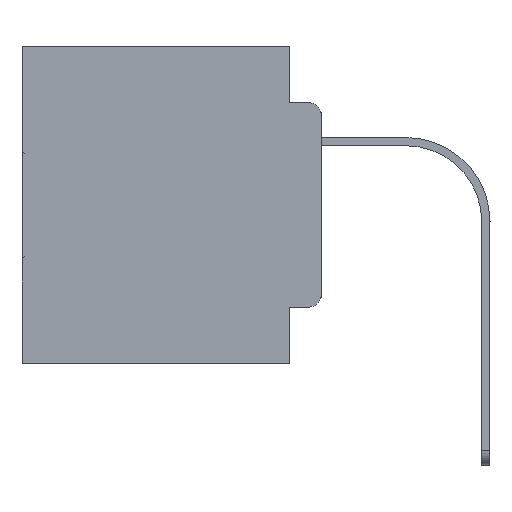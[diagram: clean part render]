
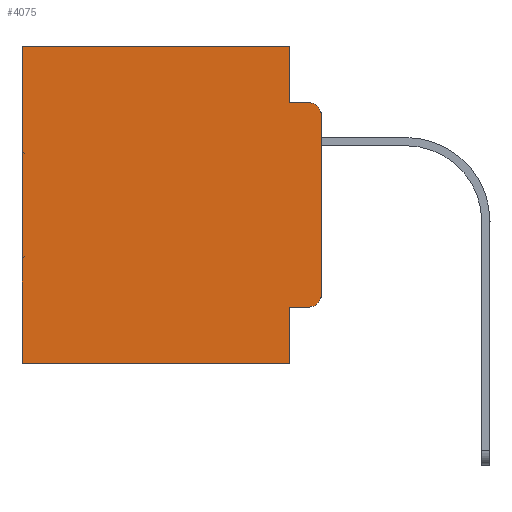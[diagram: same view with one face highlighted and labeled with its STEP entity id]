
A CAD part, left-side view. The second image highlights one B-rep face of the part: STEP entity #4075.
In plain terms, the highlighted planar face has unit normal (-1, 0, 0).
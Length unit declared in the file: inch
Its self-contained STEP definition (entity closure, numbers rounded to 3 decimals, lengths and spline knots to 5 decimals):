
#538 = VERTEX_POINT ( 'NONE', #17069 ) ;
#594 = CARTESIAN_POINT ( 'NONE',  ( 0.298, 0.473, 0. ) ) ;
#929 = DIRECTION ( 'NONE',  ( 0., 0., -1. ) ) ;
#1005 = CARTESIAN_POINT ( 'NONE',  ( 0.298, 0., 0. ) ) ;
#1598 = EDGE_CURVE ( 'NONE', #16262, #1641, #28964, .T. ) ;
#1641 = VERTEX_POINT ( 'NONE', #12351 ) ;
#2139 = LINE ( 'NONE', #21336, #22587 ) ;
#3368 = DIRECTION ( 'NONE',  ( 1., 0., 0. ) ) ;
#3558 = ORIENTED_EDGE ( 'NONE', *, *, #11707, .F. ) ;
#3778 = ORIENTED_EDGE ( 'NONE', *, *, #1598, .F. ) ;
#4075 = ADVANCED_FACE ( 'NONE', ( #20603 ), #30549, .F. ) ;
#4396 = CARTESIAN_POINT ( 'NONE',  ( 0.298, 0.051, 0. ) ) ;
#4466 = VERTEX_POINT ( 'NONE', #18658 ) ;
#6388 = EDGE_CURVE ( 'NONE', #16262, #13022, #28228, .T. ) ;
#6582 = CARTESIAN_POINT ( 'NONE',  ( 0.298, 0., -0.1085 ) ) ;
#8537 = CARTESIAN_POINT ( 'NONE',  ( 0.298, 0.051, 0. ) ) ;
#8723 = ORIENTED_EDGE ( 'NONE', *, *, #19751, .T. ) ;
#8855 = CARTESIAN_POINT ( 'NONE',  ( 0.298, 0., 0. ) ) ;
#9914 = VECTOR ( 'NONE', #22390, 39.37008 ) ;
#10277 = DIRECTION ( 'NONE',  ( 0., 0., -1. ) ) ;
#10423 = DIRECTION ( 'NONE',  ( -1., 0., 0. ) ) ;
#10648 = ORIENTED_EDGE ( 'NONE', *, *, #12283, .F. ) ;
#10711 = LINE ( 'NONE', #594, #16738 ) ;
#10853 = CARTESIAN_POINT ( 'NONE',  ( 0.298, 0., 0. ) ) ;
#11054 = CARTESIAN_POINT ( 'NONE',  ( 0.298, 0.02, -0.1085 ) ) ;
#11199 = CARTESIAN_POINT ( 'NONE',  ( 0.298, 0.473, 0. ) ) ;
#11707 = EDGE_CURVE ( 'NONE', #1641, #31300, #23032, .T. ) ;
#11749 = ORIENTED_EDGE ( 'NONE', *, *, #12856, .T. ) ;
#11909 = ORIENTED_EDGE ( 'NONE', *, *, #29803, .F. ) ;
#12055 = ORIENTED_EDGE ( 'NONE', *, *, #15059, .T. ) ;
#12086 = DIRECTION ( 'NONE',  ( 0., 1., 0. ) ) ;
#12283 = EDGE_CURVE ( 'NONE', #4466, #26132, #13297, .T. ) ;
#12351 = CARTESIAN_POINT ( 'NONE',  ( 0.298, 0.051, -0.0885 ) ) ;
#12856 = EDGE_CURVE ( 'NONE', #13022, #26415, #10711, .T. ) ;
#13017 = CARTESIAN_POINT ( 'NONE',  ( 0.298, 0.02, -0.0885 ) ) ;
#13022 = VERTEX_POINT ( 'NONE', #11199 ) ;
#13297 = LINE ( 'NONE', #8537, #20169 ) ;
#14974 = ORIENTED_EDGE ( 'NONE', *, *, #29296, .T. ) ;
#15059 = EDGE_CURVE ( 'NONE', #31865, #31300, #25568, .T. ) ;
#15273 = CARTESIAN_POINT ( 'NONE',  ( 0.298, 0.051, -0.0885 ) ) ;
#16262 = VERTEX_POINT ( 'NONE', #4396 ) ;
#16738 = VECTOR ( 'NONE', #20138, 39.37008 ) ;
#17069 = CARTESIAN_POINT ( 'NONE',  ( 0.298, 0., -0.3915 ) ) ;
#17195 = CARTESIAN_POINT ( 'NONE',  ( 0.298, 0.051, 0. ) ) ;
#18249 = DIRECTION ( 'NONE',  ( 0., 0., -1. ) ) ;
#18477 = DIRECTION ( 'NONE',  ( 0., 0., -1. ) ) ;
#18566 = DIRECTION ( 'NONE',  ( 0., 0., -1. ) ) ;
#18658 = CARTESIAN_POINT ( 'NONE',  ( 0.298, 0.051, -0.4115 ) ) ;
#18780 = DIRECTION ( 'NONE',  ( 0., 1., 0. ) ) ;
#19317 = DIRECTION ( 'NONE',  ( 0., 0., -1. ) ) ;
#19751 = EDGE_CURVE ( 'NONE', #4466, #31774, #29927, .T. ) ;
#20138 = DIRECTION ( 'NONE',  ( 0., 0., -1. ) ) ;
#20169 = VECTOR ( 'NONE', #18477, 39.37008 ) ;
#20555 = VECTOR ( 'NONE', #29755, 39.37008 ) ;
#20603 = FACE_OUTER_BOUND ( 'NONE', #21703, .T. ) ;
#20965 = DIRECTION ( 'NONE',  ( -1., 0., 0. ) ) ;
#21018 = VECTOR ( 'NONE', #18780, 39.37008 ) ;
#21336 = CARTESIAN_POINT ( 'NONE',  ( 0.298, 0., -0.5 ) ) ;
#21703 = EDGE_LOOP ( 'NONE', ( #27954, #12055, #3558, #3778, #28477, #11749, #11909, #10648, #8723, #14974 ) ) ;
#21880 = AXIS2_PLACEMENT_3D ( 'NONE', #25393, #10423, #10277 ) ;
#22253 = CARTESIAN_POINT ( 'NONE',  ( 0.298, 0.051, -0.4115 ) ) ;
#22390 = DIRECTION ( 'NONE',  ( 0., -1., 0. ) ) ;
#22587 = VECTOR ( 'NONE', #12086, 39.37008 ) ;
#23032 = LINE ( 'NONE', #15273, #9914 ) ;
#24361 = EDGE_CURVE ( 'NONE', #31865, #538, #30945, .T. ) ;
#24461 = CARTESIAN_POINT ( 'NONE',  ( 0.298, 0.051, -0.5 ) ) ;
#25013 = CIRCLE ( 'NONE', #21880, 0.02 ) ;
#25393 = CARTESIAN_POINT ( 'NONE',  ( 0.298, 0.02, -0.3915 ) ) ;
#25568 = CIRCLE ( 'NONE', #29744, 0.02 ) ;
#26132 = VERTEX_POINT ( 'NONE', #24461 ) ;
#26415 = VERTEX_POINT ( 'NONE', #27401 ) ;
#27120 = CARTESIAN_POINT ( 'NONE',  ( 0.298, 0.02, -0.4115 ) ) ;
#27401 = CARTESIAN_POINT ( 'NONE',  ( 0.298, 0.473, -0.5 ) ) ;
#27688 = VECTOR ( 'NONE', #18249, 39.37008 ) ;
#27954 = ORIENTED_EDGE ( 'NONE', *, *, #24361, .F. ) ;
#28228 = LINE ( 'NONE', #8855, #21018 ) ;
#28477 = ORIENTED_EDGE ( 'NONE', *, *, #6388, .T. ) ;
#28819 = AXIS2_PLACEMENT_3D ( 'NONE', #10853, #3368, #929 ) ;
#28964 = LINE ( 'NONE', #17195, #31840 ) ;
#29296 = EDGE_CURVE ( 'NONE', #31774, #538, #25013, .T. ) ;
#29744 = AXIS2_PLACEMENT_3D ( 'NONE', #11054, #20965, #18566 ) ;
#29755 = DIRECTION ( 'NONE',  ( 0., -1., 0. ) ) ;
#29803 = EDGE_CURVE ( 'NONE', #26132, #26415, #2139, .T. ) ;
#29927 = LINE ( 'NONE', #22253, #20555 ) ;
#30549 = PLANE ( 'NONE',  #28819 ) ;
#30945 = LINE ( 'NONE', #1005, #27688 ) ;
#31300 = VERTEX_POINT ( 'NONE', #13017 ) ;
#31774 = VERTEX_POINT ( 'NONE', #27120 ) ;
#31840 = VECTOR ( 'NONE', #19317, 39.37008 ) ;
#31865 = VERTEX_POINT ( 'NONE', #6582 ) ;
